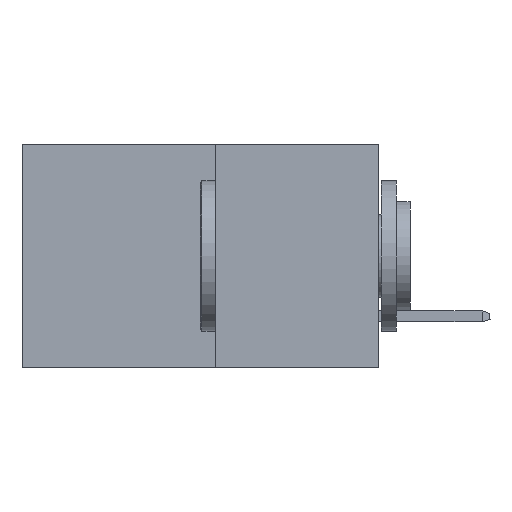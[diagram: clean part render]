
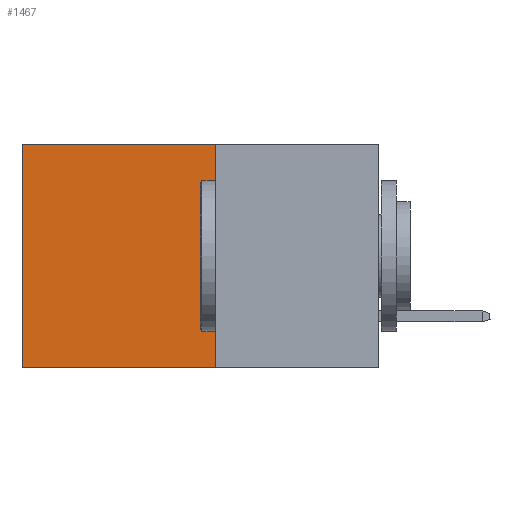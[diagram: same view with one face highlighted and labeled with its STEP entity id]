
A CAD part, left-side view. The second image highlights one B-rep face of the part: STEP entity #1467.
In plain terms, the highlighted planar face has unit normal (-1, 0, 0).
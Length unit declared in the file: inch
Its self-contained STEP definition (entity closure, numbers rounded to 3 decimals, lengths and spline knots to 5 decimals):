
#244 = LINE ( 'NONE', #12875, #3106 ) ;
#305 = EDGE_CURVE ( 'NONE', #14341, #3742, #7994, .T. ) ;
#447 = CARTESIAN_POINT ( 'NONE',  ( 0.277, 0.27, -0.37 ) ) ;
#650 = CARTESIAN_POINT ( 'NONE',  ( 0.277, 0.27, -0.37 ) ) ;
#1160 = EDGE_CURVE ( 'NONE', #2188, #3742, #7755, .T. ) ;
#1467 = ADVANCED_FACE ( 'NONE', ( #8885 ), #4971, .F. ) ;
#2110 = CARTESIAN_POINT ( 'NONE',  ( 0.277, 0.27, -0.37 ) ) ;
#2188 = VERTEX_POINT ( 'NONE', #2605 ) ;
#2605 = CARTESIAN_POINT ( 'NONE',  ( 0.277, 0.27, -0.37 ) ) ;
#3106 = VECTOR ( 'NONE', #12401, 39.37008 ) ;
#3332 = DIRECTION ( 'NONE',  ( 0., 0., -1. ) ) ;
#3354 = ORIENTED_EDGE ( 'NONE', *, *, #1160, .F. ) ;
#3742 = VERTEX_POINT ( 'NONE', #12180 ) ;
#4224 = CARTESIAN_POINT ( 'NONE',  ( 0.277, 0.27, 0. ) ) ;
#4768 = VECTOR ( 'NONE', #14136, 39.37008 ) ;
#4971 = PLANE ( 'NONE',  #8201 ) ;
#5379 = EDGE_CURVE ( 'NONE', #9549, #14341, #244, .T. ) ;
#6692 = DIRECTION ( 'NONE',  ( 0., 0., -1. ) ) ;
#7755 = LINE ( 'NONE', #650, #13841 ) ;
#7994 = LINE ( 'NONE', #14387, #4768 ) ;
#8201 = AXIS2_PLACEMENT_3D ( 'NONE', #447, #13985, #6692 ) ;
#8814 = CARTESIAN_POINT ( 'NONE',  ( 0.277, 0.59, 0. ) ) ;
#8885 = FACE_OUTER_BOUND ( 'NONE', #11417, .T. ) ;
#9549 = VERTEX_POINT ( 'NONE', #4224 ) ;
#10313 = DIRECTION ( 'NONE',  ( 0., 1., 0. ) ) ;
#10821 = VECTOR ( 'NONE', #3332, 39.37008 ) ;
#10934 = ORIENTED_EDGE ( 'NONE', *, *, #5379, .T. ) ;
#11417 = EDGE_LOOP ( 'NONE', ( #13191, #3354, #13394, #10934 ) ) ;
#12180 = CARTESIAN_POINT ( 'NONE',  ( 0.277, 0.59, -0.37 ) ) ;
#12401 = DIRECTION ( 'NONE',  ( 0., 1., 0. ) ) ;
#12875 = CARTESIAN_POINT ( 'NONE',  ( 0.277, 0.27, 0. ) ) ;
#13191 = ORIENTED_EDGE ( 'NONE', *, *, #305, .T. ) ;
#13394 = ORIENTED_EDGE ( 'NONE', *, *, #13970, .F. ) ;
#13841 = VECTOR ( 'NONE', #10313, 39.37008 ) ;
#13970 = EDGE_CURVE ( 'NONE', #9549, #2188, #14031, .T. ) ;
#13985 = DIRECTION ( 'NONE',  ( 1., 0., 0. ) ) ;
#14031 = LINE ( 'NONE', #2110, #10821 ) ;
#14136 = DIRECTION ( 'NONE',  ( 0., 0., -1. ) ) ;
#14341 = VERTEX_POINT ( 'NONE', #8814 ) ;
#14387 = CARTESIAN_POINT ( 'NONE',  ( 0.277, 0.59, -0.37 ) ) ;
